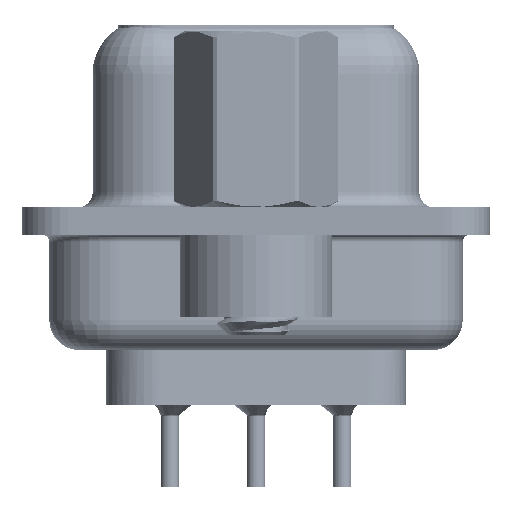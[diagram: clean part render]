
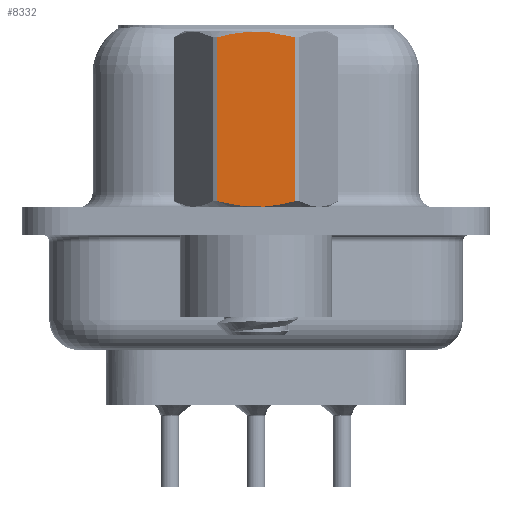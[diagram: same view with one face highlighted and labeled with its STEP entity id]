
A CAD part, left-side view. The second image highlights one B-rep face of the part: STEP entity #8332.
In plain terms, the highlighted planar face has unit normal (-1, 0, 0).
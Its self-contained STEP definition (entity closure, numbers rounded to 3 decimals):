
#1450 = EDGE_CURVE ( 'NONE', #20413, #19456, #26109, .T. ) ;
#2278 = CARTESIAN_POINT ( 'NONE',  ( -2.381, 1.273, 0.652 ) ) ;
#4646 = CARTESIAN_POINT ( 'NONE',  ( -2.381, 1.273, 6.048 ) ) ;
#5982 = ORIENTED_EDGE ( 'NONE', *, *, #33156, .T. ) ;
#6955 = DIRECTION ( 'NONE',  ( 0., -1., 0. ) ) ;
#7567 = AXIS2_PLACEMENT_3D ( 'NONE', #45687, #27795, #6955 ) ;
#8332 = ADVANCED_FACE ( 'NONE', ( #35994 ), #31259, .T. ) ;
#9640 = VECTOR ( 'NONE', #27598, 1000. ) ;
#9762 = CARTESIAN_POINT ( 'NONE',  ( -2.381, -0.432, 6.215 ) ) ;
#11426 = VERTEX_POINT ( 'NONE', #21300 ) ;
#13355 = CARTESIAN_POINT ( 'NONE',  ( -2.381, 0.215, 6.232 ) ) ;
#16942 = CARTESIAN_POINT ( 'NONE',  ( -2.381, 0.853, 6.151 ) ) ;
#16984 = B_SPLINE_CURVE_WITH_KNOTS ( 'NONE', 3,
 ( #27632, #24028, #31248, #9762, #34899, #13355, #38509, #16942, #42086, #20545 ),
 .UNSPECIFIED., .F., .F.,
 ( 4, 2, 2, 2, 4 ),
 ( 0.001, 0.002, 0.002, 0.003, 0.004 ),
 .UNSPECIFIED. ) ;
#19142 = LINE ( 'NONE', #45324, #9640 ) ;
#19456 = VERTEX_POINT ( 'NONE', #34862 ) ;
#20413 = VERTEX_POINT ( 'NONE', #2278 ) ;
#20545 = CARTESIAN_POINT ( 'NONE',  ( -2.381, 1.273, 6.048 ) ) ;
#21300 = CARTESIAN_POINT ( 'NONE',  ( -2.381, -1.273, 6.048 ) ) ;
#22325 = CARTESIAN_POINT ( 'NONE',  ( -2.381, 1.273, 0.652 ) ) ;
#24028 = CARTESIAN_POINT ( 'NONE',  ( -2.381, -1.066, 6.104 ) ) ;
#24424 = CARTESIAN_POINT ( 'NONE',  ( -2.381, 0.853, 0.549 ) ) ;
#26093 = CARTESIAN_POINT ( 'NONE',  ( -2.381, -1.066, 0.596 ) ) ;
#26109 = B_SPLINE_CURVE_WITH_KNOTS ( 'NONE', 3,
 ( #22325, #31810, #24424, #26869, #26730, #26572, #26413, #26250, #26093, #35777 ),
 .UNSPECIFIED., .F., .F.,
 ( 4, 2, 2, 2, 4 ),
 ( 0.003, 0.003, 0.004, 0.004, 0.005 ),
 .UNSPECIFIED. ) ;
#26250 = CARTESIAN_POINT ( 'NONE',  ( -2.381, -0.858, 0.55 ) ) ;
#26413 = CARTESIAN_POINT ( 'NONE',  ( -2.381, -0.432, 0.485 ) ) ;
#26572 = CARTESIAN_POINT ( 'NONE',  ( -2.381, -0.215, 0.468 ) ) ;
#26730 = CARTESIAN_POINT ( 'NONE',  ( -2.381, 0.215, 0.468 ) ) ;
#26869 = CARTESIAN_POINT ( 'NONE',  ( -2.381, 0.428, 0.485 ) ) ;
#27598 = DIRECTION ( 'NONE',  ( 0., 0., 1. ) ) ;
#27632 = CARTESIAN_POINT ( 'NONE',  ( -2.381, -1.273, 6.048 ) ) ;
#27795 = DIRECTION ( 'NONE',  ( -1., 0., 0. ) ) ;
#29532 = ORIENTED_EDGE ( 'NONE', *, *, #1450, .T. ) ;
#31248 = CARTESIAN_POINT ( 'NONE',  ( -2.381, -0.858, 6.15 ) ) ;
#31259 = PLANE ( 'NONE',  #7567 ) ;
#31810 = CARTESIAN_POINT ( 'NONE',  ( -2.381, 1.065, 0.596 ) ) ;
#31987 = CARTESIAN_POINT ( 'NONE',  ( -2.381, 1.273, 3.792 ) ) ;
#32242 = EDGE_LOOP ( 'NONE', ( #29532, #44041, #36452, #5982 ) ) ;
#33156 = EDGE_CURVE ( 'NONE', #36774, #20413, #44745, .T. ) ;
#34862 = CARTESIAN_POINT ( 'NONE',  ( -2.381, -1.273, 0.652 ) ) ;
#34899 = CARTESIAN_POINT ( 'NONE',  ( -2.381, -0.215, 6.232 ) ) ;
#35635 = DIRECTION ( 'NONE',  ( 0., 0., -1. ) ) ;
#35777 = CARTESIAN_POINT ( 'NONE',  ( -2.381, -1.273, 0.652 ) ) ;
#35994 = FACE_OUTER_BOUND ( 'NONE', #32242, .T. ) ;
#36452 = ORIENTED_EDGE ( 'NONE', *, *, #46064, .T. ) ;
#36774 = VERTEX_POINT ( 'NONE', #4646 ) ;
#37982 = EDGE_CURVE ( 'NONE', #19456, #11426, #19142, .T. ) ;
#38509 = CARTESIAN_POINT ( 'NONE',  ( -2.381, 0.428, 6.215 ) ) ;
#42086 = CARTESIAN_POINT ( 'NONE',  ( -2.381, 1.065, 6.104 ) ) ;
#43636 = VECTOR ( 'NONE', #35635, 1000. ) ;
#44041 = ORIENTED_EDGE ( 'NONE', *, *, #37982, .T. ) ;
#44745 = LINE ( 'NONE', #31987, #43636 ) ;
#45324 = CARTESIAN_POINT ( 'NONE',  ( -2.381, -1.273, 3.792 ) ) ;
#45687 = CARTESIAN_POINT ( 'NONE',  ( -2.381, 1.375, -3.75 ) ) ;
#46064 = EDGE_CURVE ( 'NONE', #11426, #36774, #16984, .T. ) ;
